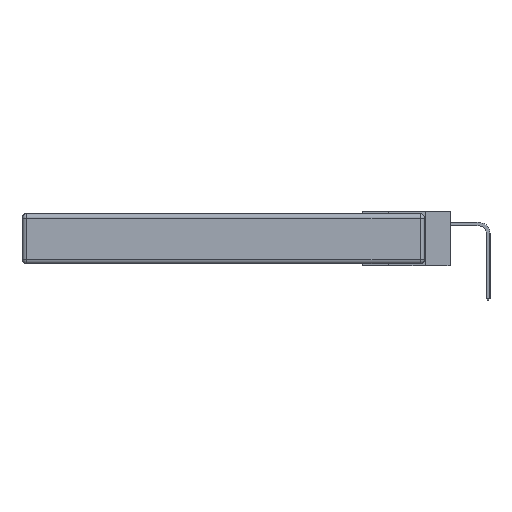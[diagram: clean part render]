
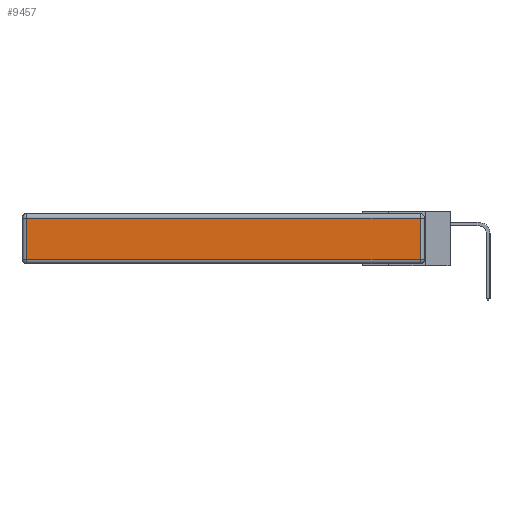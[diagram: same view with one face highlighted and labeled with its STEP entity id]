
A CAD part, left-side view. The second image highlights one B-rep face of the part: STEP entity #9457.
In plain terms, the highlighted planar face has unit normal (-1, 0, 0).
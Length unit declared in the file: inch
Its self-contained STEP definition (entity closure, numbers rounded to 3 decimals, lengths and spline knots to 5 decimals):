
#602 = AXIS2_PLACEMENT_3D ( 'NONE', #15813, #24658, #2505 ) ;
#1657 = DIRECTION ( 'NONE',  ( 0., 0., -1. ) ) ;
#2412 = EDGE_CURVE ( 'NONE', #24365, #21236, #14521, .T. ) ;
#2505 = DIRECTION ( 'NONE',  ( 0., 0., 1. ) ) ;
#2688 = CARTESIAN_POINT ( 'NONE',  ( 0., 2.72, -0.03 ) ) ;
#3447 = DIRECTION ( 'NONE',  ( 0., 0., 1. ) ) ;
#3546 = CARTESIAN_POINT ( 'NONE',  ( 0., 0.03, -0.313 ) ) ;
#4782 = FACE_OUTER_BOUND ( 'NONE', #6053, .T. ) ;
#5705 = CARTESIAN_POINT ( 'NONE',  ( 0., 0., -0.313 ) ) ;
#6053 = EDGE_LOOP ( 'NONE', ( #12031, #8541, #12583, #27074 ) ) ;
#6798 = CARTESIAN_POINT ( 'NONE',  ( 0., 0.03, -0.343 ) ) ;
#7572 = EDGE_CURVE ( 'NONE', #21236, #16002, #12870, .T. ) ;
#8167 = DIRECTION ( 'NONE',  ( 0., -1., 0. ) ) ;
#8541 = ORIENTED_EDGE ( 'NONE', *, *, #2412, .T. ) ;
#8746 = VERTEX_POINT ( 'NONE', #21616 ) ;
#9302 = PLANE ( 'NONE',  #602 ) ;
#9457 = ADVANCED_FACE ( 'NONE', ( #4782 ), #9302, .T. ) ;
#9689 = VECTOR ( 'NONE', #19611, 39.37008 ) ;
#12031 = ORIENTED_EDGE ( 'NONE', *, *, #13547, .T. ) ;
#12583 = ORIENTED_EDGE ( 'NONE', *, *, #7572, .T. ) ;
#12870 = LINE ( 'NONE', #26449, #9689 ) ;
#13547 = EDGE_CURVE ( 'NONE', #8746, #24365, #20235, .T. ) ;
#13648 = VECTOR ( 'NONE', #8167, 39.37008 ) ;
#13831 = VECTOR ( 'NONE', #3447, 39.37008 ) ;
#14521 = LINE ( 'NONE', #6798, #13831 ) ;
#15813 = CARTESIAN_POINT ( 'NONE',  ( 0., 0., -0.343 ) ) ;
#15827 = EDGE_CURVE ( 'NONE', #16002, #8746, #28353, .T. ) ;
#16002 = VERTEX_POINT ( 'NONE', #2688 ) ;
#17044 = CARTESIAN_POINT ( 'NONE',  ( 0., 2.72, -0.343 ) ) ;
#19611 = DIRECTION ( 'NONE',  ( 0., 1., 0. ) ) ;
#20235 = LINE ( 'NONE', #5705, #13648 ) ;
#21236 = VERTEX_POINT ( 'NONE', #27746 ) ;
#21449 = VECTOR ( 'NONE', #1657, 39.37008 ) ;
#21616 = CARTESIAN_POINT ( 'NONE',  ( 0., 2.72, -0.313 ) ) ;
#24365 = VERTEX_POINT ( 'NONE', #3546 ) ;
#24658 = DIRECTION ( 'NONE',  ( -1., 0., 0. ) ) ;
#26449 = CARTESIAN_POINT ( 'NONE',  ( 0., 2.75, -0.03 ) ) ;
#27074 = ORIENTED_EDGE ( 'NONE', *, *, #15827, .T. ) ;
#27746 = CARTESIAN_POINT ( 'NONE',  ( 0., 0.03, -0.03 ) ) ;
#28353 = LINE ( 'NONE', #17044, #21449 ) ;
